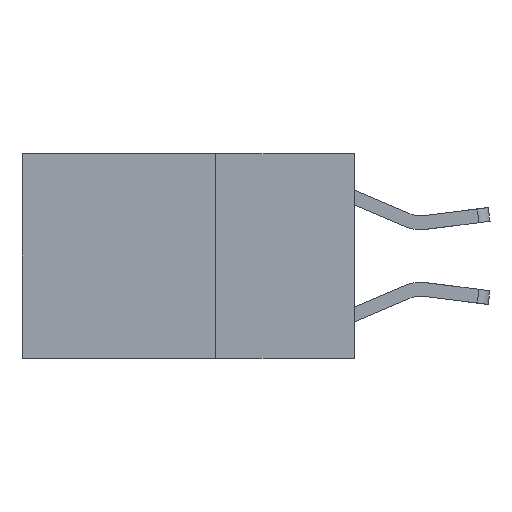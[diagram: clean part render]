
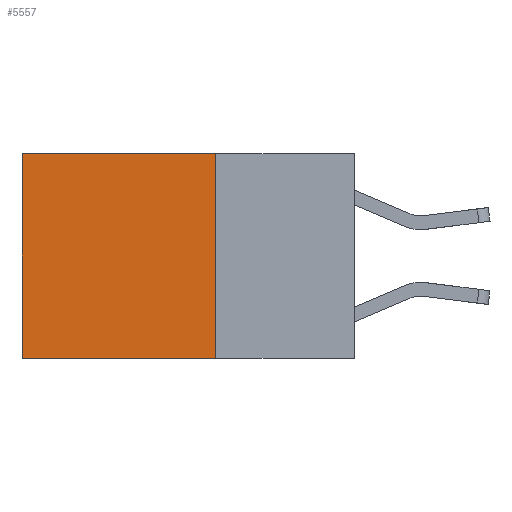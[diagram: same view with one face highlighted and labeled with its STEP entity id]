
A CAD part, left-side view. The second image highlights one B-rep face of the part: STEP entity #5557.
In plain terms, the highlighted planar face has unit normal (-1, 0, 0).
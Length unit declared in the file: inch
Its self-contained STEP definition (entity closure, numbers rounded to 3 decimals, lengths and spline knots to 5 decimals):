
#956 = EDGE_LOOP ( 'NONE', ( #1776, #6545, #7150, #5475 ) ) ;
#1440 = VERTEX_POINT ( 'NONE', #1954 ) ;
#1498 = VERTEX_POINT ( 'NONE', #5099 ) ;
#1678 = VECTOR ( 'NONE', #1714, 39.37008 ) ;
#1714 = DIRECTION ( 'NONE',  ( 0., 1., 0. ) ) ;
#1776 = ORIENTED_EDGE ( 'NONE', *, *, #6638, .T. ) ;
#1880 = LINE ( 'NONE', #4841, #5726 ) ;
#1954 = CARTESIAN_POINT ( 'NONE',  ( 0.2625, 0.6, 0. ) ) ;
#2973 = EDGE_CURVE ( 'NONE', #3089, #5828, #3112, .T. ) ;
#3013 = DIRECTION ( 'NONE',  ( 0., 1., 0. ) ) ;
#3089 = VERTEX_POINT ( 'NONE', #4144 ) ;
#3112 = LINE ( 'NONE', #8020, #6677 ) ;
#3257 = DIRECTION ( 'NONE',  ( 0., 0., -1. ) ) ;
#3316 = EDGE_CURVE ( 'NONE', #3089, #1440, #7924, .T. ) ;
#4144 = CARTESIAN_POINT ( 'NONE',  ( 0.2625, 0.25, 0. ) ) ;
#4415 = CARTESIAN_POINT ( 'NONE',  ( 0.2625, 0.25, -0.37 ) ) ;
#4605 = CARTESIAN_POINT ( 'NONE',  ( 0.2625, 0.25, 0. ) ) ;
#4672 = DIRECTION ( 'NONE',  ( 0., 0., -1. ) ) ;
#4841 = CARTESIAN_POINT ( 'NONE',  ( 0.2625, 0.6, 0. ) ) ;
#5005 = CARTESIAN_POINT ( 'NONE',  ( 0.2625, 0.25, -0.37 ) ) ;
#5099 = CARTESIAN_POINT ( 'NONE',  ( 0.2625, 0.6, -0.37 ) ) ;
#5324 = DIRECTION ( 'NONE',  ( 1., 0., 0. ) ) ;
#5438 = EDGE_CURVE ( 'NONE', #5828, #1498, #8567, .T. ) ;
#5475 = ORIENTED_EDGE ( 'NONE', *, *, #3316, .T. ) ;
#5557 = ADVANCED_FACE ( 'NONE', ( #8059 ), #6604, .F. ) ;
#5726 = VECTOR ( 'NONE', #4672, 39.37008 ) ;
#5828 = VERTEX_POINT ( 'NONE', #4415 ) ;
#5879 = VECTOR ( 'NONE', #3013, 39.37008 ) ;
#6002 = CARTESIAN_POINT ( 'NONE',  ( 0.2625, 0.25, 0. ) ) ;
#6545 = ORIENTED_EDGE ( 'NONE', *, *, #5438, .F. ) ;
#6604 = PLANE ( 'NONE',  #6615 ) ;
#6615 = AXIS2_PLACEMENT_3D ( 'NONE', #4605, #5324, #8831 ) ;
#6638 = EDGE_CURVE ( 'NONE', #1440, #1498, #1880, .T. ) ;
#6677 = VECTOR ( 'NONE', #3257, 39.37008 ) ;
#7150 = ORIENTED_EDGE ( 'NONE', *, *, #2973, .F. ) ;
#7924 = LINE ( 'NONE', #6002, #1678 ) ;
#8020 = CARTESIAN_POINT ( 'NONE',  ( 0.2625, 0.25, 0. ) ) ;
#8059 = FACE_OUTER_BOUND ( 'NONE', #956, .T. ) ;
#8567 = LINE ( 'NONE', #5005, #5879 ) ;
#8831 = DIRECTION ( 'NONE',  ( 0., 0., -1. ) ) ;
